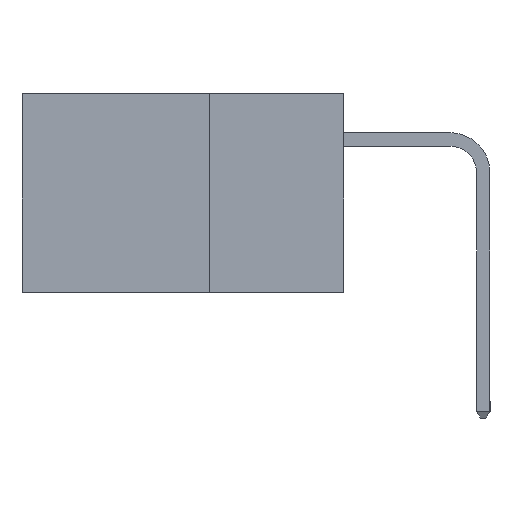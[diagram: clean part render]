
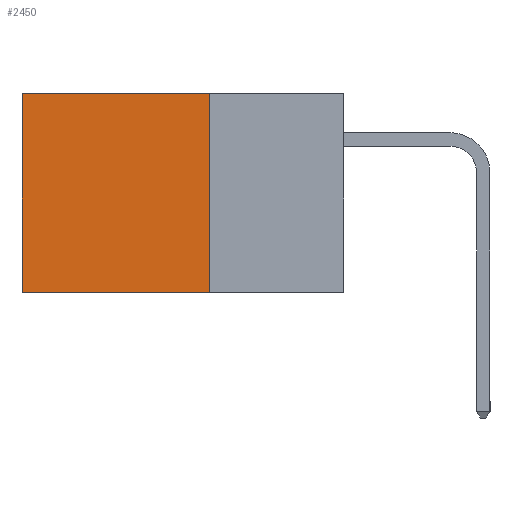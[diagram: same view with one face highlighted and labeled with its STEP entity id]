
A CAD part, left-side view. The second image highlights one B-rep face of the part: STEP entity #2450.
In plain terms, the highlighted planar face has unit normal (-1, 0, 0).
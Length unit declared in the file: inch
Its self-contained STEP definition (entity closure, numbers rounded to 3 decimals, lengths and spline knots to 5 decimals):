
#118 = LINE ( 'NONE', #12926, #741 ) ;
#741 = VECTOR ( 'NONE', #13178, 39.37008 ) ;
#823 = AXIS2_PLACEMENT_3D ( 'NONE', #20735, #5905, #18423 ) ;
#2322 = CARTESIAN_POINT ( 'NONE',  ( 0.2615, 0.6, -0.37 ) ) ;
#2450 = ADVANCED_FACE ( 'NONE', ( #16551 ), #21013, .F. ) ;
#2494 = ORIENTED_EDGE ( 'NONE', *, *, #17059, .F. ) ;
#3415 = LINE ( 'NONE', #4622, #23673 ) ;
#3547 = VERTEX_POINT ( 'NONE', #5070 ) ;
#4109 = DIRECTION ( 'NONE',  ( 0., 0., -1. ) ) ;
#4622 = CARTESIAN_POINT ( 'NONE',  ( 0.2615, 0.6, -0.37 ) ) ;
#5070 = CARTESIAN_POINT ( 'NONE',  ( 0.2615, 0.6, 0. ) ) ;
#5905 = DIRECTION ( 'NONE',  ( 1., 0., 0. ) ) ;
#6026 = VECTOR ( 'NONE', #23861, 39.37008 ) ;
#7959 = DIRECTION ( 'NONE',  ( 0., 0., -1. ) ) ;
#8320 = EDGE_CURVE ( 'NONE', #18444, #3547, #118, .T. ) ;
#9677 = LINE ( 'NONE', #17816, #19593 ) ;
#10131 = ORIENTED_EDGE ( 'NONE', *, *, #8320, .T. ) ;
#10224 = ORIENTED_EDGE ( 'NONE', *, *, #12914, .T. ) ;
#12914 = EDGE_CURVE ( 'NONE', #3547, #17734, #3415, .T. ) ;
#12926 = CARTESIAN_POINT ( 'NONE',  ( 0.2615, 0.25, 0. ) ) ;
#13178 = DIRECTION ( 'NONE',  ( 0., 1., 0. ) ) ;
#13552 = CARTESIAN_POINT ( 'NONE',  ( 0.2615, 0.25, -0.37 ) ) ;
#16551 = FACE_OUTER_BOUND ( 'NONE', #23145, .T. ) ;
#17059 = EDGE_CURVE ( 'NONE', #18444, #23523, #9677, .T. ) ;
#17734 = VERTEX_POINT ( 'NONE', #2322 ) ;
#17816 = CARTESIAN_POINT ( 'NONE',  ( 0.2615, 0.25, -0.37 ) ) ;
#18423 = DIRECTION ( 'NONE',  ( 0., 0., -1. ) ) ;
#18444 = VERTEX_POINT ( 'NONE', #23705 ) ;
#19593 = VECTOR ( 'NONE', #7959, 39.37008 ) ;
#20735 = CARTESIAN_POINT ( 'NONE',  ( 0.2615, 0.25, -0.37 ) ) ;
#21013 = PLANE ( 'NONE',  #823 ) ;
#21946 = CARTESIAN_POINT ( 'NONE',  ( 0.2615, 0.25, -0.37 ) ) ;
#22317 = LINE ( 'NONE', #21946, #6026 ) ;
#23145 = EDGE_LOOP ( 'NONE', ( #10224, #24685, #2494, #10131 ) ) ;
#23523 = VERTEX_POINT ( 'NONE', #13552 ) ;
#23673 = VECTOR ( 'NONE', #4109, 39.37008 ) ;
#23681 = EDGE_CURVE ( 'NONE', #23523, #17734, #22317, .T. ) ;
#23705 = CARTESIAN_POINT ( 'NONE',  ( 0.2615, 0.25, 0. ) ) ;
#23861 = DIRECTION ( 'NONE',  ( 0., 1., 0. ) ) ;
#24685 = ORIENTED_EDGE ( 'NONE', *, *, #23681, .F. ) ;
